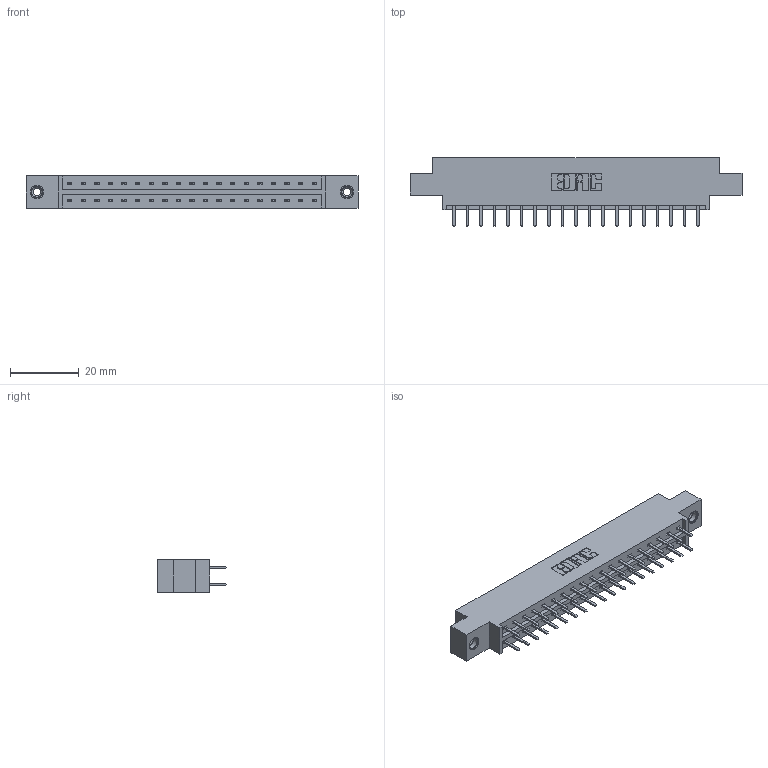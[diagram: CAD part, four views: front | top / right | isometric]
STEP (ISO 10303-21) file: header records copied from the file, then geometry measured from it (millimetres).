
FILE_DESCRIPTION (( 'STEP AP203' ), '1' );
FILE_NAME ('833-038-520-808.STEP', '2020-06-03T06:30:30', ( '' ), ( '' ), 'SwSTEP 2.0', 'SolidWorks 2020', '' );
FILE_SCHEMA (( 'CONFIG_CONTROL_DESIGN' ));
Length unit declared in the file: inch
Products named in the file (4): 833-038-520-808; 345-292-001_345-293-120; 345-250-001_345-250-003-102; 833 Part_Offset - .156 Dia - TI
Assembly tree (41 placements, depth 2):
  833-038-520-808
    833 Part_Offset - .156 Dia - TI
    345-292-001_345-293-120  x38
    345-250-001_345-250-003-102  x2
Bounding box: 96.82 x 20.02 x 9.4 mm (x, y, z)
Volume: 9419.2 mm3; surface area: 11087 mm2
Topology: 41 solids, 41 shells, 2306 faces, 6653 edges, 4326 vertices
Faces by surface type: plane 1550, cylinder 740, cone 12, torus 4
Entity records: 16630 total; most frequent: CARTESIAN_POINT 2781, ORIENTED_EDGE 2698, DIRECTION 2435, EDGE_CURVE 1349, LINE 1197, VECTOR 1197, VERTEX_POINT 892, AXIS2_PLACEMENT_3D 619
